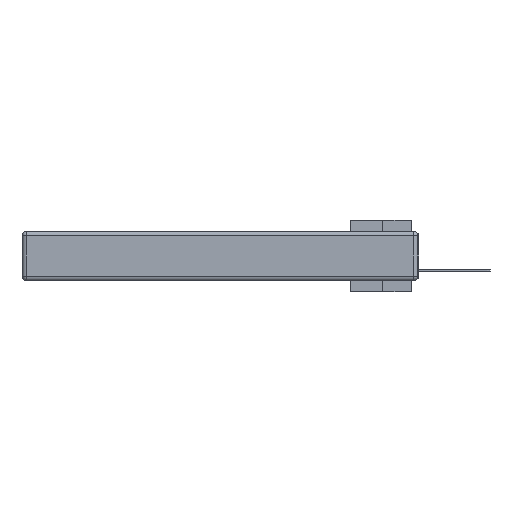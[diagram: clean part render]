
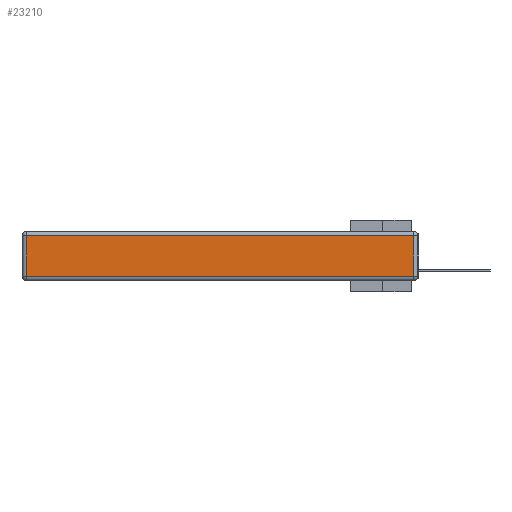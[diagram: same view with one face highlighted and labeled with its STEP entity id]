
A CAD part, left-side view. The second image highlights one B-rep face of the part: STEP entity #23210.
In plain terms, the highlighted planar face has unit normal (-1, 0, 0).
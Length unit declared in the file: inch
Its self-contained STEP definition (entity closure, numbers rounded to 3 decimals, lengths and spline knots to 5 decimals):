
#2992 = CARTESIAN_POINT ( 'NONE',  ( 0., 2.72, -0.343 ) ) ;
#3632 = EDGE_CURVE ( 'NONE', #21112, #22684, #13841, .T. ) ;
#3840 = CARTESIAN_POINT ( 'NONE',  ( 0., 0.03, -0.03 ) ) ;
#4365 = VECTOR ( 'NONE', #12046, 39.37008 ) ;
#5809 = FACE_OUTER_BOUND ( 'NONE', #17312, .T. ) ;
#6369 = PLANE ( 'NONE',  #31495 ) ;
#7713 = ORIENTED_EDGE ( 'NONE', *, *, #3632, .T. ) ;
#10006 = LINE ( 'NONE', #14186, #24248 ) ;
#11447 = CARTESIAN_POINT ( 'NONE',  ( 0., 0., -0.343 ) ) ;
#12046 = DIRECTION ( 'NONE',  ( 0., 0., 1. ) ) ;
#13841 = LINE ( 'NONE', #2992, #24892 ) ;
#14186 = CARTESIAN_POINT ( 'NONE',  ( 0., 2.75, -0.03 ) ) ;
#14534 = EDGE_CURVE ( 'NONE', #21044, #17394, #24903, .T. ) ;
#16543 = VECTOR ( 'NONE', #30358, 39.37008 ) ;
#17312 = EDGE_LOOP ( 'NONE', ( #19034, #25229, #25010, #7713 ) ) ;
#17394 = VERTEX_POINT ( 'NONE', #3840 ) ;
#19034 = ORIENTED_EDGE ( 'NONE', *, *, #22294, .T. ) ;
#21044 = VERTEX_POINT ( 'NONE', #24777 ) ;
#21112 = VERTEX_POINT ( 'NONE', #24567 ) ;
#22294 = EDGE_CURVE ( 'NONE', #22684, #21044, #28453, .T. ) ;
#22684 = VERTEX_POINT ( 'NONE', #31660 ) ;
#23210 = ADVANCED_FACE ( 'NONE', ( #5809 ), #6369, .T. ) ;
#24248 = VECTOR ( 'NONE', #28935, 39.37008 ) ;
#24567 = CARTESIAN_POINT ( 'NONE',  ( 0., 2.72, -0.03 ) ) ;
#24777 = CARTESIAN_POINT ( 'NONE',  ( 0., 0.03, -0.313 ) ) ;
#24892 = VECTOR ( 'NONE', #28122, 39.37008 ) ;
#24903 = LINE ( 'NONE', #31915, #4365 ) ;
#25010 = ORIENTED_EDGE ( 'NONE', *, *, #28778, .T. ) ;
#25229 = ORIENTED_EDGE ( 'NONE', *, *, #14534, .T. ) ;
#28122 = DIRECTION ( 'NONE',  ( 0., 0., -1. ) ) ;
#28453 = LINE ( 'NONE', #30020, #16543 ) ;
#28778 = EDGE_CURVE ( 'NONE', #17394, #21112, #10006, .T. ) ;
#28935 = DIRECTION ( 'NONE',  ( 0., 1., 0. ) ) ;
#29070 = DIRECTION ( 'NONE',  ( -1., 0., 0. ) ) ;
#30020 = CARTESIAN_POINT ( 'NONE',  ( 0., 0., -0.313 ) ) ;
#30358 = DIRECTION ( 'NONE',  ( 0., -1., 0. ) ) ;
#31495 = AXIS2_PLACEMENT_3D ( 'NONE', #11447, #29070, #31619 ) ;
#31619 = DIRECTION ( 'NONE',  ( 0., 0., 1. ) ) ;
#31660 = CARTESIAN_POINT ( 'NONE',  ( 0., 2.72, -0.313 ) ) ;
#31915 = CARTESIAN_POINT ( 'NONE',  ( 0., 0.03, -0.343 ) ) ;
